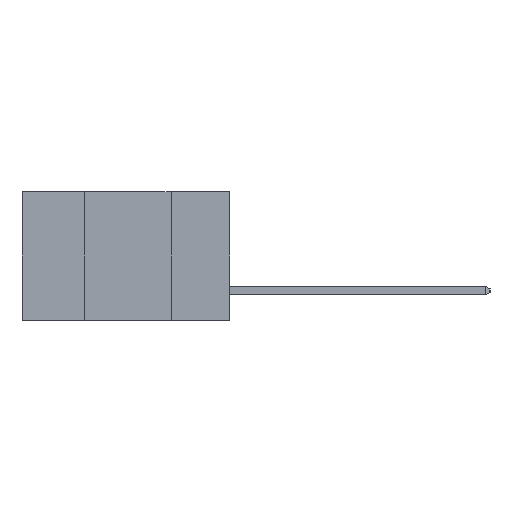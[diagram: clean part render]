
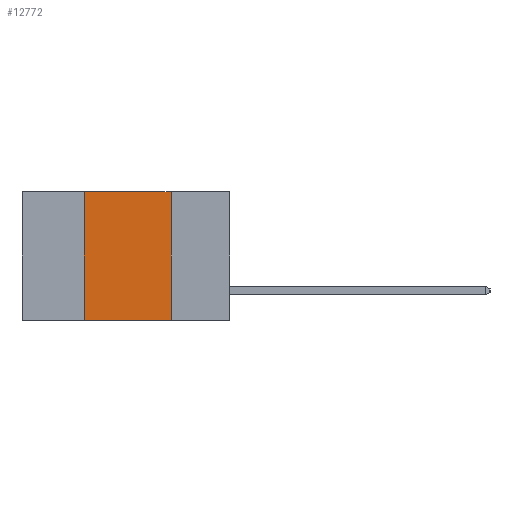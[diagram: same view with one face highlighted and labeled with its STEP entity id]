
A CAD part, left-side view. The second image highlights one B-rep face of the part: STEP entity #12772.
In plain terms, the highlighted planar face has unit normal (-1, 0, 0).
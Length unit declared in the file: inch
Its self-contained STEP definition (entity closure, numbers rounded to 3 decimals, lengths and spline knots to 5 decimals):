
#419 = DIRECTION ( 'NONE',  ( 0., -1., 0. ) ) ;
#768 = ORIENTED_EDGE ( 'NONE', *, *, #4585, .F. ) ;
#908 = CARTESIAN_POINT ( 'NONE',  ( 0., 0.42, 0. ) ) ;
#1441 = LINE ( 'NONE', #16748, #19687 ) ;
#1728 = VECTOR ( 'NONE', #6191, 39.37008 ) ;
#2405 = ORIENTED_EDGE ( 'NONE', *, *, #4388, .F. ) ;
#2742 = VERTEX_POINT ( 'NONE', #3902 ) ;
#3832 = LINE ( 'NONE', #9248, #7954 ) ;
#3902 = CARTESIAN_POINT ( 'NONE',  ( 0., 0.17, 0. ) ) ;
#4388 = EDGE_CURVE ( 'NONE', #5168, #2742, #1441, .T. ) ;
#4585 = EDGE_CURVE ( 'NONE', #2742, #9162, #6484, .T. ) ;
#4754 = LINE ( 'NONE', #12855, #13334 ) ;
#5168 = VERTEX_POINT ( 'NONE', #908 ) ;
#6090 = DIRECTION ( 'NONE',  ( 0., -1., 0. ) ) ;
#6191 = DIRECTION ( 'NONE',  ( 0., 0., -1. ) ) ;
#6484 = LINE ( 'NONE', #6491, #1728 ) ;
#6491 = CARTESIAN_POINT ( 'NONE',  ( 0., 0.17, 0. ) ) ;
#7189 = ORIENTED_EDGE ( 'NONE', *, *, #12990, .F. ) ;
#7954 = VECTOR ( 'NONE', #419, 39.37008 ) ;
#8396 = VERTEX_POINT ( 'NONE', #14592 ) ;
#9162 = VERTEX_POINT ( 'NONE', #19636 ) ;
#9248 = CARTESIAN_POINT ( 'NONE',  ( 0., 0.6, -0.37 ) ) ;
#9296 = ORIENTED_EDGE ( 'NONE', *, *, #19413, .T. ) ;
#10168 = EDGE_LOOP ( 'NONE', ( #768, #2405, #7189, #9296 ) ) ;
#10819 = AXIS2_PLACEMENT_3D ( 'NONE', #16750, #16506, #16438 ) ;
#12601 = DIRECTION ( 'NONE',  ( 0., 0., 1. ) ) ;
#12772 = ADVANCED_FACE ( 'NONE', ( #18542 ), #16766, .F. ) ;
#12855 = CARTESIAN_POINT ( 'NONE',  ( 0., 0.42, 0. ) ) ;
#12990 = EDGE_CURVE ( 'NONE', #8396, #5168, #4754, .T. ) ;
#13334 = VECTOR ( 'NONE', #12601, 39.37008 ) ;
#14592 = CARTESIAN_POINT ( 'NONE',  ( 0., 0.42, -0.37 ) ) ;
#16438 = DIRECTION ( 'NONE',  ( 0., 0., -1. ) ) ;
#16506 = DIRECTION ( 'NONE',  ( 1., 0., 0. ) ) ;
#16748 = CARTESIAN_POINT ( 'NONE',  ( 0., 0.6, 0. ) ) ;
#16750 = CARTESIAN_POINT ( 'NONE',  ( 0., 0.6, 0. ) ) ;
#16766 = PLANE ( 'NONE',  #10819 ) ;
#18542 = FACE_OUTER_BOUND ( 'NONE', #10168, .T. ) ;
#19413 = EDGE_CURVE ( 'NONE', #8396, #9162, #3832, .T. ) ;
#19636 = CARTESIAN_POINT ( 'NONE',  ( 0., 0.17, -0.37 ) ) ;
#19687 = VECTOR ( 'NONE', #6090, 39.37008 ) ;
